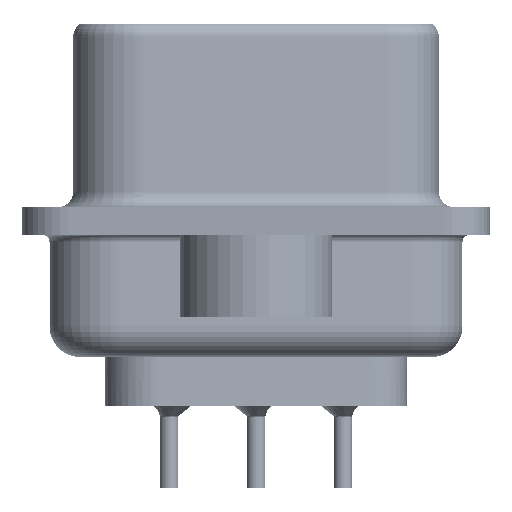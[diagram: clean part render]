
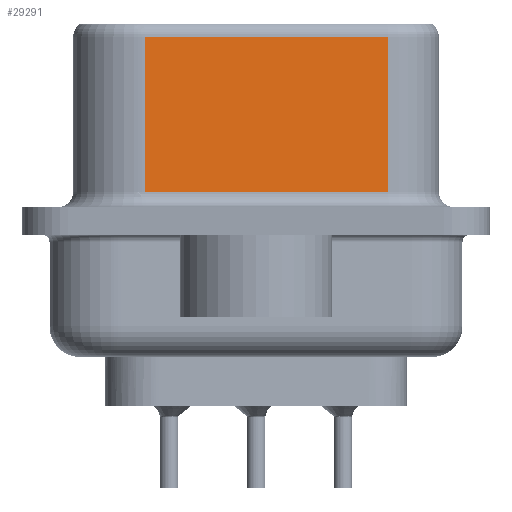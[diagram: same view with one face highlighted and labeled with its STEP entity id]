
A CAD part, left-side view. The second image highlights one B-rep face of the part: STEP entity #29291.
In plain terms, the highlighted planar face has unit normal (-0.985, -0.174, 0).
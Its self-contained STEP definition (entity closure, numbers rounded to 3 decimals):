
#593 = CARTESIAN_POINT ( 'NONE',  ( 5.132, -4.322, 6.52 ) ) ;
#1839 = EDGE_LOOP ( 'NONE', ( #6330, #25113, #4107, #23101 ) ) ;
#2963 = VECTOR ( 'NONE', #30876, 1000. ) ;
#3446 = LINE ( 'NONE', #27733, #17362 ) ;
#4107 = ORIENTED_EDGE ( 'NONE', *, *, #8695, .T. ) ;
#4694 = EDGE_CURVE ( 'NONE', #7239, #9652, #20122, .T. ) ;
#5216 = AXIS2_PLACEMENT_3D ( 'NONE', #593, #6314, #25405 ) ;
#6314 = DIRECTION ( 'NONE',  ( 0.985, 0.174, 0. ) ) ;
#6330 = ORIENTED_EDGE ( 'NONE', *, *, #4694, .F. ) ;
#7239 = VERTEX_POINT ( 'NONE', #21299 ) ;
#8187 = EDGE_CURVE ( 'NONE', #7239, #12826, #3446, .T. ) ;
#8695 = EDGE_CURVE ( 'NONE', #12826, #32835, #31860, .T. ) ;
#9652 = VERTEX_POINT ( 'NONE', #20294 ) ;
#12826 = VERTEX_POINT ( 'NONE', #25106 ) ;
#12912 = EDGE_CURVE ( 'NONE', #32835, #9652, #24885, .T. ) ;
#14135 = CARTESIAN_POINT ( 'NONE',  ( 3.73, 3.628, 6.52 ) ) ;
#14585 = PLANE ( 'NONE',  #5216 ) ;
#16243 = CARTESIAN_POINT ( 'NONE',  ( 5.132, -4.322, 6.52 ) ) ;
#16847 = DIRECTION ( 'NONE',  ( 0., 0., -1. ) ) ;
#17362 = VECTOR ( 'NONE', #27616, 1000. ) ;
#20122 = LINE ( 'NONE', #16243, #33595 ) ;
#20294 = CARTESIAN_POINT ( 'NONE',  ( 5.132, -4.322, 0.95 ) ) ;
#21299 = CARTESIAN_POINT ( 'NONE',  ( 5.132, -4.322, 6.02 ) ) ;
#21564 = FACE_OUTER_BOUND ( 'NONE', #1839, .T. ) ;
#23101 = ORIENTED_EDGE ( 'NONE', *, *, #12912, .T. ) ;
#24885 = LINE ( 'NONE', #25460, #2963 ) ;
#25106 = CARTESIAN_POINT ( 'NONE',  ( 3.73, 3.628, 6.02 ) ) ;
#25113 = ORIENTED_EDGE ( 'NONE', *, *, #8187, .T. ) ;
#25405 = DIRECTION ( 'NONE',  ( -0.174, 0.985, 0. ) ) ;
#25460 = CARTESIAN_POINT ( 'NONE',  ( 5.132, -4.322, 0.95 ) ) ;
#27616 = DIRECTION ( 'NONE',  ( -0.174, 0.985, 0. ) ) ;
#27733 = CARTESIAN_POINT ( 'NONE',  ( 5.132, -4.322, 6.02 ) ) ;
#29291 = ADVANCED_FACE ( 'NONE', ( #21564 ), #14585, .F. ) ;
#30876 = DIRECTION ( 'NONE',  ( 0.174, -0.985, 0. ) ) ;
#30993 = VECTOR ( 'NONE', #16847, 1000. ) ;
#31860 = LINE ( 'NONE', #14135, #30993 ) ;
#32835 = VERTEX_POINT ( 'NONE', #33466 ) ;
#33466 = CARTESIAN_POINT ( 'NONE',  ( 3.73, 3.628, 0.95 ) ) ;
#33595 = VECTOR ( 'NONE', #35081, 1000. ) ;
#35081 = DIRECTION ( 'NONE',  ( 0., 0., -1. ) ) ;
